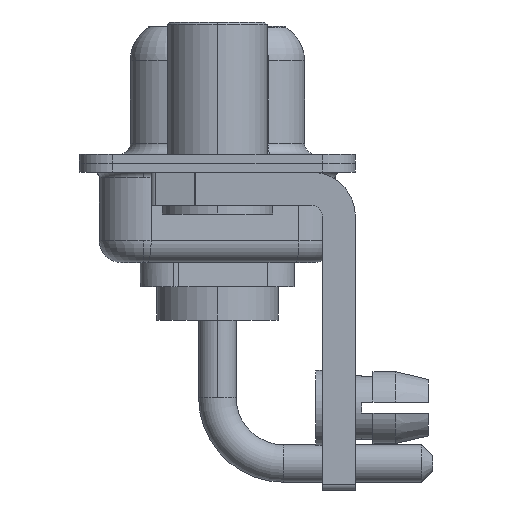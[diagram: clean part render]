
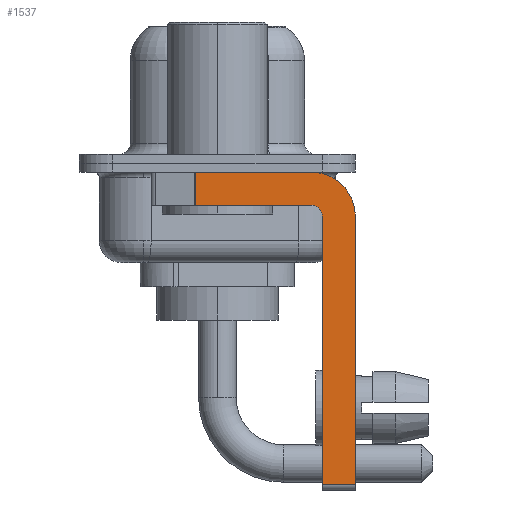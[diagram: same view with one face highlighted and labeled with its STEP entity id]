
A CAD part, left-side view. The second image highlights one B-rep face of the part: STEP entity #1537.
In plain terms, the highlighted planar face has unit normal (-1, 0, 0).
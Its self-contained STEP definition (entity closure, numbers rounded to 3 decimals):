
#69 = ORIENTED_EDGE ( 'NONE', *, *, #11975, .F. ) ;
#135 = EDGE_CURVE ( 'NONE', #2969, #8568, #6799, .T. ) ;
#522 = CARTESIAN_POINT ( 'NONE',  ( -2.9, 3., -0.4 ) ) ;
#546 = EDGE_CURVE ( 'NONE', #3387, #6813, #5382, .T. ) ;
#824 = CARTESIAN_POINT ( 'NONE',  ( -2.9, -4.25, -0.4 ) ) ;
#1351 = DIRECTION ( 'NONE',  ( 1., 0., 0. ) ) ;
#1537 = ADVANCED_FACE ( 'NONE', ( #2410 ), #6108, .F. ) ;
#1895 = CARTESIAN_POINT ( 'NONE',  ( -2.9, -4.25, -2.4 ) ) ;
#1933 = DIRECTION ( 'NONE',  ( 0., 0., -1. ) ) ;
#2410 = FACE_OUTER_BOUND ( 'NONE', #13349, .T. ) ;
#2411 = VERTEX_POINT ( 'NONE', #5309 ) ;
#2778 = CARTESIAN_POINT ( 'NONE',  ( -2.9, 0.978, -1.9 ) ) ;
#2969 = VERTEX_POINT ( 'NONE', #824 ) ;
#2973 = LINE ( 'NONE', #522, #12413 ) ;
#3329 = CARTESIAN_POINT ( 'NONE',  ( -2.9, -4.75, -14.55 ) ) ;
#3387 = VERTEX_POINT ( 'NONE', #3329 ) ;
#3409 = DIRECTION ( 'NONE',  ( 0., 1., 0. ) ) ;
#3416 = EDGE_CURVE ( 'NONE', #2411, #11351, #13295, .T. ) ;
#3552 = CARTESIAN_POINT ( 'NONE',  ( -2.9, -4.25, -2.4 ) ) ;
#3788 = LINE ( 'NONE', #13838, #12289 ) ;
#4076 = VECTOR ( 'NONE', #3409, 1000. ) ;
#4295 = DIRECTION ( 'NONE',  ( 0., -1., 0. ) ) ;
#4299 = VECTOR ( 'NONE', #13335, 1000. ) ;
#4764 = ORIENTED_EDGE ( 'NONE', *, *, #12813, .F. ) ;
#5309 = CARTESIAN_POINT ( 'NONE',  ( -2.9, -4.25, -1.9 ) ) ;
#5382 = LINE ( 'NONE', #10550, #13118 ) ;
#5703 = CARTESIAN_POINT ( 'NONE',  ( -2.9, -4.25, -2.4 ) ) ;
#5797 = ORIENTED_EDGE ( 'NONE', *, *, #135, .F. ) ;
#6086 = CARTESIAN_POINT ( 'NONE',  ( -2.9, -6.25, -14.55 ) ) ;
#6108 = PLANE ( 'NONE',  #14177 ) ;
#6199 = DIRECTION ( 'NONE',  ( 0., 0., -1. ) ) ;
#6767 = AXIS2_PLACEMENT_3D ( 'NONE', #5703, #15900, #13424 ) ;
#6799 = CIRCLE ( 'NONE', #9161, 2. ) ;
#6813 = VERTEX_POINT ( 'NONE', #6086 ) ;
#6933 = LINE ( 'NONE', #10701, #4299 ) ;
#7022 = ORIENTED_EDGE ( 'NONE', *, *, #10554, .F. ) ;
#7296 = ORIENTED_EDGE ( 'NONE', *, *, #546, .T. ) ;
#7481 = CARTESIAN_POINT ( 'NONE',  ( -2.9, -4.75, -2.4 ) ) ;
#8117 = VECTOR ( 'NONE', #1933, 1000. ) ;
#8198 = LINE ( 'NONE', #14197, #8117 ) ;
#8359 = CARTESIAN_POINT ( 'NONE',  ( -2.9, -4.25, -1.9 ) ) ;
#8568 = VERTEX_POINT ( 'NONE', #15546 ) ;
#9161 = AXIS2_PLACEMENT_3D ( 'NONE', #1895, #12005, #10690 ) ;
#9175 = VERTEX_POINT ( 'NONE', #11864 ) ;
#9236 = DIRECTION ( 'NONE',  ( 0., -1., 0. ) ) ;
#9536 = VERTEX_POINT ( 'NONE', #7481 ) ;
#10410 = EDGE_CURVE ( 'NONE', #9175, #2969, #2973, .T. ) ;
#10550 = CARTESIAN_POINT ( 'NONE',  ( -2.9, -4.25, -14.55 ) ) ;
#10554 = EDGE_CURVE ( 'NONE', #3387, #9536, #6933, .T. ) ;
#10690 = DIRECTION ( 'NONE',  ( 0., 0., -1. ) ) ;
#10701 = CARTESIAN_POINT ( 'NONE',  ( -2.9, -4.75, -14.8 ) ) ;
#11220 = CIRCLE ( 'NONE', #6767, 0.5 ) ;
#11351 = VERTEX_POINT ( 'NONE', #2778 ) ;
#11864 = CARTESIAN_POINT ( 'NONE',  ( -2.9, 0.978, -0.4 ) ) ;
#11975 = EDGE_CURVE ( 'NONE', #8568, #6813, #8198, .T. ) ;
#12005 = DIRECTION ( 'NONE',  ( 1., 0., 0. ) ) ;
#12090 = ORIENTED_EDGE ( 'NONE', *, *, #10410, .F. ) ;
#12102 = EDGE_CURVE ( 'NONE', #9175, #11351, #3788, .T. ) ;
#12289 = VECTOR ( 'NONE', #14592, 1000. ) ;
#12413 = VECTOR ( 'NONE', #4295, 1000. ) ;
#12813 = EDGE_CURVE ( 'NONE', #9536, #2411, #11220, .T. ) ;
#13073 = ORIENTED_EDGE ( 'NONE', *, *, #3416, .F. ) ;
#13118 = VECTOR ( 'NONE', #9236, 1000. ) ;
#13295 = LINE ( 'NONE', #8359, #4076 ) ;
#13335 = DIRECTION ( 'NONE',  ( 0., 0., 1. ) ) ;
#13349 = EDGE_LOOP ( 'NONE', ( #12090, #14714, #13073, #4764, #7022, #7296, #69, #5797 ) ) ;
#13424 = DIRECTION ( 'NONE',  ( 0., 0., 1. ) ) ;
#13838 = CARTESIAN_POINT ( 'NONE',  ( -2.9, 0.978, -1.9 ) ) ;
#14177 = AXIS2_PLACEMENT_3D ( 'NONE', #3552, #1351, #6199 ) ;
#14197 = CARTESIAN_POINT ( 'NONE',  ( -2.9, -6.25, -2.4 ) ) ;
#14592 = DIRECTION ( 'NONE',  ( 0., 0., -1. ) ) ;
#14714 = ORIENTED_EDGE ( 'NONE', *, *, #12102, .T. ) ;
#15546 = CARTESIAN_POINT ( 'NONE',  ( -2.9, -6.25, -2.4 ) ) ;
#15900 = DIRECTION ( 'NONE',  ( -1., 0., 0. ) ) ;
